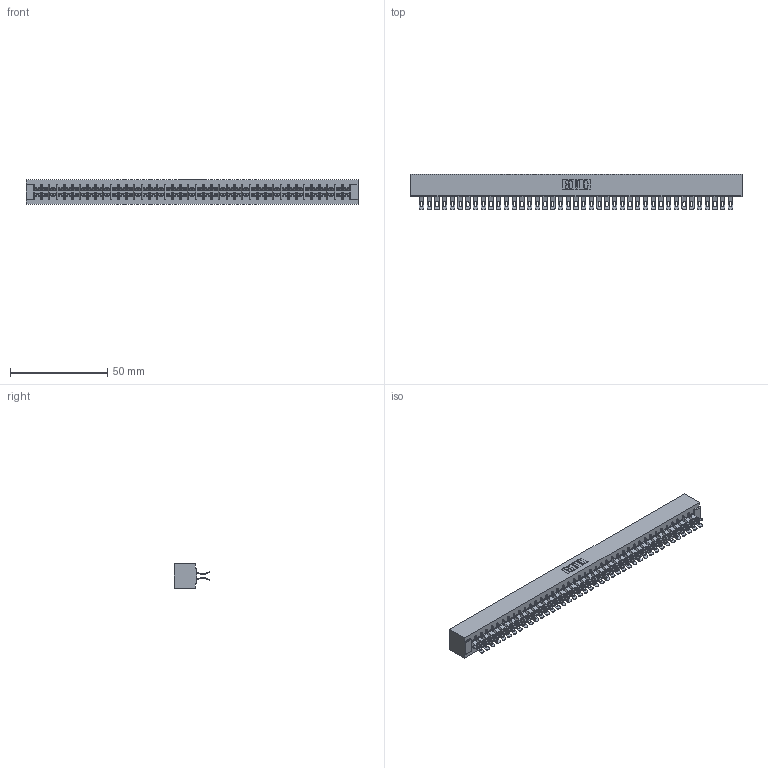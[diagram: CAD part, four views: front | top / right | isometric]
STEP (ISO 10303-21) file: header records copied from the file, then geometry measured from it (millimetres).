
FILE_DESCRIPTION (( 'STEP AP203' ), '1' );
FILE_NAME ('315-082-555-201.STEP', '2019-09-10T23:35:47', ( '' ), ( '' ), 'SwSTEP 2.0', 'SolidWorks 2016', '' );
FILE_SCHEMA (( 'CONFIG_CONTROL_DESIGN' ));
Length unit declared in the file: inch
Products named in the file (3): 315-082-555-201; 305 Part_No Mounting; 305-290-001_555
Assembly tree (83 placements, depth 2):
  315-082-555-201
    305 Part_No Mounting
    305-290-001_555  x82
Bounding box: 170.33 x 18.41 x 12.7 mm (x, y, z)
Volume: 18492.1 mm3; surface area: 25449.8 mm2
Topology: 83 solids, 83 shells, 5520 faces, 16487 edges, 10770 vertices
Faces by surface type: plane 2688, cylinder 2668, sphere 164
Entity records: 44860 total; most frequent: CARTESIAN_POINT 7439, ORIENTED_EDGE 7374, DIRECTION 7189, EDGE_CURVE 3687, LINE 2965, VECTOR 2965, VERTEX_POINT 2346, AXIS2_PLACEMENT_3D 2112
